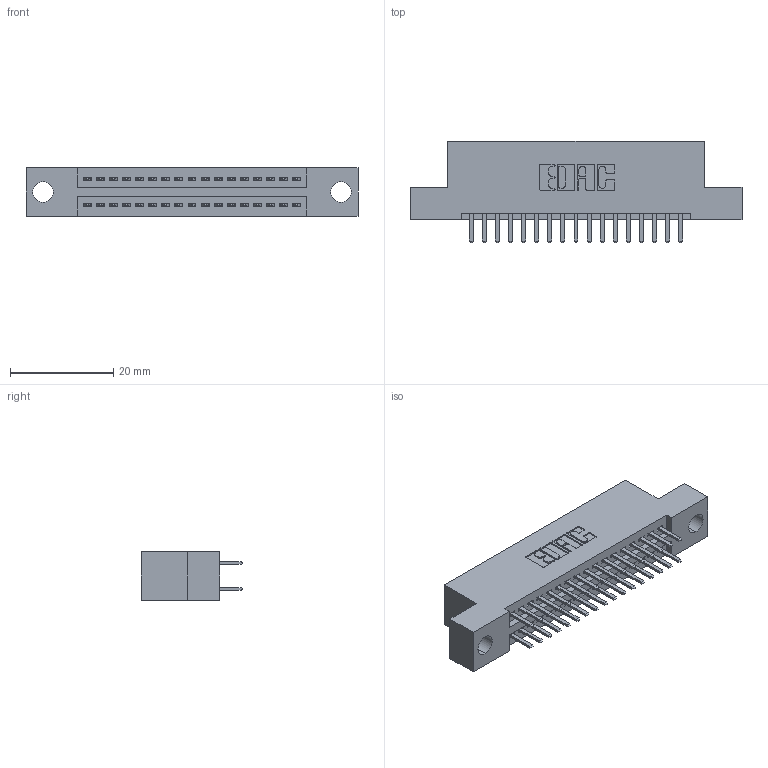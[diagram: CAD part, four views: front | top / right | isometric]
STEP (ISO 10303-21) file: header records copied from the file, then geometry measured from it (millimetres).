
FILE_DESCRIPTION (( 'STEP AP203' ), '1' );
FILE_NAME ('345-034-520-204.STEP', '2021-05-19T23:57:03', ( '' ), ( '' ), 'SwSTEP 2.0', 'SolidWorks 2020', '' );
FILE_SCHEMA (( 'CONFIG_CONTROL_DESIGN' ));
Length unit declared in the file: inch
Products named in the file (3): 345 Part_Flush Mounting Lugs - 0.156 Dia-TI; 345-292-001_345-293-120; 345-034-520-204
Assembly tree (35 placements, depth 2):
  345-034-520-204
    345 Part_Flush Mounting Lugs - 0.156 Dia-TI
    345-292-001_345-293-120  x34
Bounding box: 64.39 x 19.68 x 9.4 mm (x, y, z)
Volume: 5901.9 mm3; surface area: 8059.5 mm2
Topology: 35 solids, 35 shells, 1976 faces, 5715 edges, 3718 vertices
Faces by surface type: plane 1284, cylinder 692
Entity records: 17237 total; most frequent: CARTESIAN_POINT 2930, ORIENTED_EDGE 2850, DIRECTION 2601, EDGE_CURVE 1425, LINE 1221, VECTOR 1221, VERTEX_POINT 946, AXIS2_PLACEMENT_3D 690
